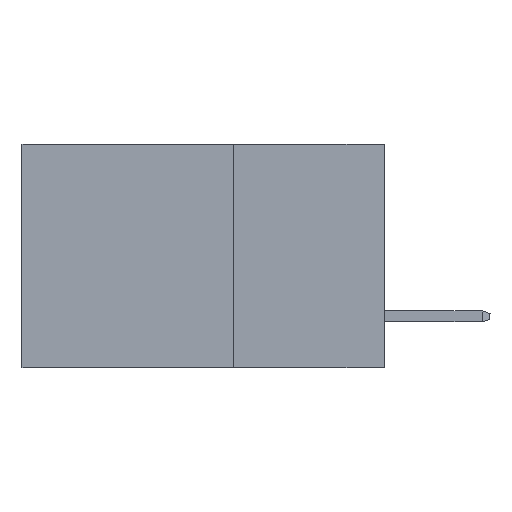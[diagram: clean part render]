
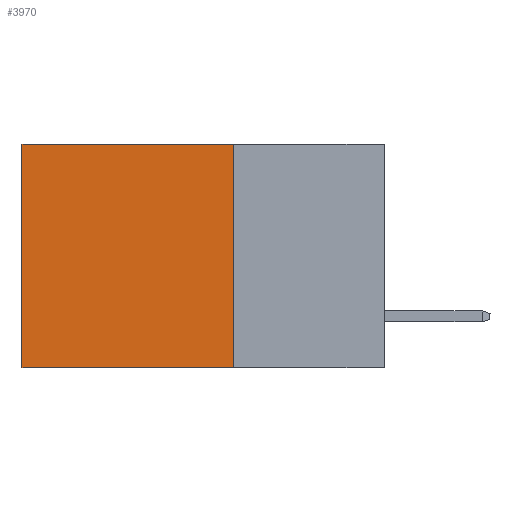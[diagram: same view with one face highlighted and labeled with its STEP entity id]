
A CAD part, left-side view. The second image highlights one B-rep face of the part: STEP entity #3970.
In plain terms, the highlighted planar face has unit normal (-1, 0, 0).
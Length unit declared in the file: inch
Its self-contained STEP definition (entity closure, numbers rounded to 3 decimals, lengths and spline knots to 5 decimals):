
#72 = LINE ( 'NONE', #12196, #9294 ) ;
#276 = VERTEX_POINT ( 'NONE', #10383 ) ;
#1565 = VECTOR ( 'NONE', #8768, 39.37008 ) ;
#1643 = ORIENTED_EDGE ( 'NONE', *, *, #4446, .T. ) ;
#1838 = DIRECTION ( 'NONE',  ( 1., 0., 0. ) ) ;
#2139 = LINE ( 'NONE', #15936, #9426 ) ;
#3405 = EDGE_LOOP ( 'NONE', ( #9527, #11414, #13722, #1643 ) ) ;
#3484 = CARTESIAN_POINT ( 'NONE',  ( 0.298, 0.25, -0.37 ) ) ;
#3623 = FACE_OUTER_BOUND ( 'NONE', #3405, .T. ) ;
#3970 = ADVANCED_FACE ( 'NONE', ( #3623 ), #11725, .F. ) ;
#4068 = LINE ( 'NONE', #12395, #1565 ) ;
#4446 = EDGE_CURVE ( 'NONE', #276, #9633, #15175, .T. ) ;
#5146 = CARTESIAN_POINT ( 'NONE',  ( 0.298, 0.6, -0.37 ) ) ;
#5630 = DIRECTION ( 'NONE',  ( 0., 0., -1. ) ) ;
#5787 = DIRECTION ( 'NONE',  ( 0., 1., 0. ) ) ;
#6062 = EDGE_CURVE ( 'NONE', #9633, #15013, #72, .T. ) ;
#7160 = EDGE_CURVE ( 'NONE', #7811, #15013, #2139, .T. ) ;
#7811 = VERTEX_POINT ( 'NONE', #3484 ) ;
#8161 = CARTESIAN_POINT ( 'NONE',  ( 0.298, 0.6, 0. ) ) ;
#8402 = CARTESIAN_POINT ( 'NONE',  ( 0.298, 0.25, 0. ) ) ;
#8756 = DIRECTION ( 'NONE',  ( 0., 0., -1. ) ) ;
#8768 = DIRECTION ( 'NONE',  ( 0., 0., -1. ) ) ;
#9294 = VECTOR ( 'NONE', #8756, 39.37008 ) ;
#9426 = VECTOR ( 'NONE', #11273, 39.37008 ) ;
#9527 = ORIENTED_EDGE ( 'NONE', *, *, #6062, .T. ) ;
#9633 = VERTEX_POINT ( 'NONE', #8161 ) ;
#10383 = CARTESIAN_POINT ( 'NONE',  ( 0.298, 0.25, 0. ) ) ;
#10520 = AXIS2_PLACEMENT_3D ( 'NONE', #14050, #1838, #5630 ) ;
#11273 = DIRECTION ( 'NONE',  ( 0., 1., 0. ) ) ;
#11414 = ORIENTED_EDGE ( 'NONE', *, *, #7160, .F. ) ;
#11725 = PLANE ( 'NONE',  #10520 ) ;
#12196 = CARTESIAN_POINT ( 'NONE',  ( 0.298, 0.6, 0. ) ) ;
#12395 = CARTESIAN_POINT ( 'NONE',  ( 0.298, 0.25, 0. ) ) ;
#12466 = EDGE_CURVE ( 'NONE', #276, #7811, #4068, .T. ) ;
#13722 = ORIENTED_EDGE ( 'NONE', *, *, #12466, .F. ) ;
#14050 = CARTESIAN_POINT ( 'NONE',  ( 0.298, 0.25, 0. ) ) ;
#15013 = VERTEX_POINT ( 'NONE', #5146 ) ;
#15175 = LINE ( 'NONE', #8402, #15735 ) ;
#15735 = VECTOR ( 'NONE', #5787, 39.37008 ) ;
#15936 = CARTESIAN_POINT ( 'NONE',  ( 0.298, 0.25, -0.37 ) ) ;
